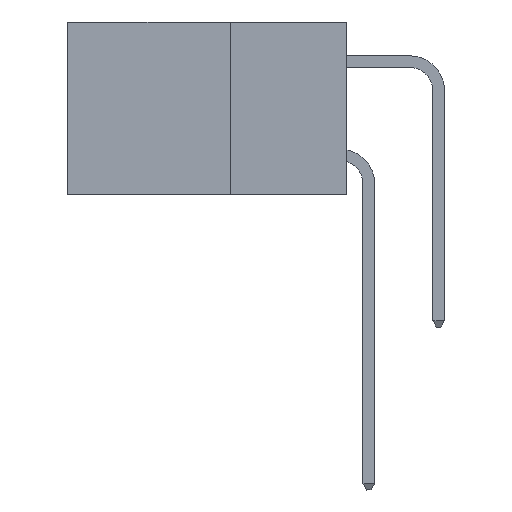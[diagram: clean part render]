
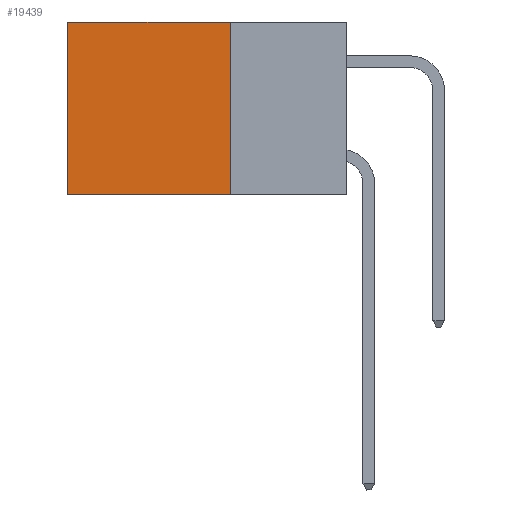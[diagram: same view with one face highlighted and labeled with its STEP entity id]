
A CAD part, left-side view. The second image highlights one B-rep face of the part: STEP entity #19439.
In plain terms, the highlighted planar face has unit normal (-1, 0, 0).
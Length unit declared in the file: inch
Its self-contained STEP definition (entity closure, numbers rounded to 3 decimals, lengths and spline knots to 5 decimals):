
#92 = DIRECTION ( 'NONE',  ( 0., 0., -1. ) ) ;
#230 = ORIENTED_EDGE ( 'NONE', *, *, #18520, .F. ) ;
#395 = CARTESIAN_POINT ( 'NONE',  ( 0.2875, 0.6, 0. ) ) ;
#514 = LINE ( 'NONE', #395, #12466 ) ;
#605 = DIRECTION ( 'NONE',  ( 0., 0., -1. ) ) ;
#654 = CARTESIAN_POINT ( 'NONE',  ( 0.2875, 0.25, -0.37 ) ) ;
#963 = DIRECTION ( 'NONE',  ( 0., 1., 0. ) ) ;
#1615 = EDGE_CURVE ( 'NONE', #2577, #14766, #21396, .T. ) ;
#2577 = VERTEX_POINT ( 'NONE', #7640 ) ;
#2769 = CARTESIAN_POINT ( 'NONE',  ( 0.2875, 0.25, 0. ) ) ;
#4199 = EDGE_LOOP ( 'NONE', ( #10239, #21927, #230, #14206 ) ) ;
#4911 = VECTOR ( 'NONE', #15563, 39.37008 ) ;
#5103 = VECTOR ( 'NONE', #19187, 39.37008 ) ;
#5331 = PLANE ( 'NONE',  #18798 ) ;
#5667 = CARTESIAN_POINT ( 'NONE',  ( 0.2875, 0.25, 0. ) ) ;
#6352 = EDGE_CURVE ( 'NONE', #13099, #12865, #21201, .T. ) ;
#7101 = CARTESIAN_POINT ( 'NONE',  ( 0.2875, 0.25, -0.37 ) ) ;
#7126 = DIRECTION ( 'NONE',  ( 1., 0., 0. ) ) ;
#7640 = CARTESIAN_POINT ( 'NONE',  ( 0.2875, 0.25, 0. ) ) ;
#10239 = ORIENTED_EDGE ( 'NONE', *, *, #20960, .T. ) ;
#12466 = VECTOR ( 'NONE', #605, 39.37008 ) ;
#12865 = VERTEX_POINT ( 'NONE', #14489 ) ;
#13099 = VERTEX_POINT ( 'NONE', #7101 ) ;
#14206 = ORIENTED_EDGE ( 'NONE', *, *, #1615, .T. ) ;
#14489 = CARTESIAN_POINT ( 'NONE',  ( 0.2875, 0.6, -0.37 ) ) ;
#14766 = VERTEX_POINT ( 'NONE', #18377 ) ;
#15563 = DIRECTION ( 'NONE',  ( 0., 0., -1. ) ) ;
#17154 = FACE_OUTER_BOUND ( 'NONE', #4199, .T. ) ;
#18377 = CARTESIAN_POINT ( 'NONE',  ( 0.2875, 0.6, 0. ) ) ;
#18520 = EDGE_CURVE ( 'NONE', #2577, #13099, #20828, .T. ) ;
#18798 = AXIS2_PLACEMENT_3D ( 'NONE', #5667, #7126, #92 ) ;
#18898 = VECTOR ( 'NONE', #963, 39.37008 ) ;
#19187 = DIRECTION ( 'NONE',  ( 0., 1., 0. ) ) ;
#19439 = ADVANCED_FACE ( 'NONE', ( #17154 ), #5331, .F. ) ;
#20828 = LINE ( 'NONE', #22037, #4911 ) ;
#20960 = EDGE_CURVE ( 'NONE', #14766, #12865, #514, .T. ) ;
#21201 = LINE ( 'NONE', #654, #5103 ) ;
#21396 = LINE ( 'NONE', #2769, #18898 ) ;
#21927 = ORIENTED_EDGE ( 'NONE', *, *, #6352, .F. ) ;
#22037 = CARTESIAN_POINT ( 'NONE',  ( 0.2875, 0.25, 0. ) ) ;
